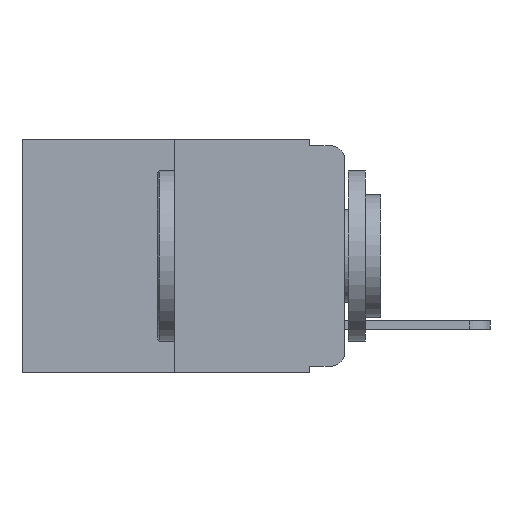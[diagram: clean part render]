
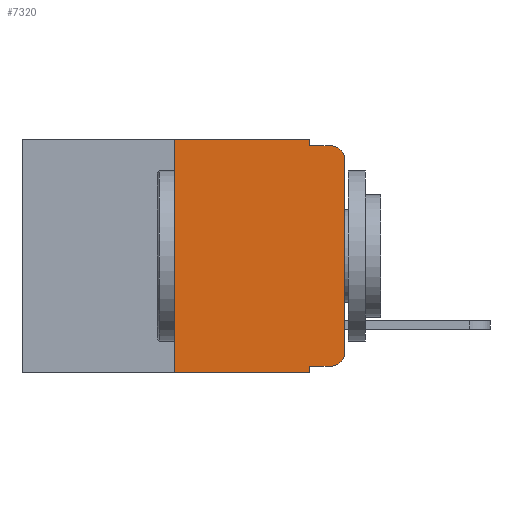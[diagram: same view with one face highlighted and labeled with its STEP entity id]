
A CAD part, left-side view. The second image highlights one B-rep face of the part: STEP entity #7320.
In plain terms, the highlighted planar face has unit normal (-1, 0, 0).
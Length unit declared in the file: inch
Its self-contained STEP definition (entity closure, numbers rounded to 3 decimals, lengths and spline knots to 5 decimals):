
#87 = VECTOR ( 'NONE', #11603, 39.37008 ) ;
#90 = LINE ( 'NONE', #11860, #87 ) ;
#93 = VERTEX_POINT ( 'NONE', #8918 ) ;
#112 = VECTOR ( 'NONE', #10868, 39.37008 ) ;
#142 = VECTOR ( 'NONE', #11367, 39.37008 ) ;
#178 = LINE ( 'NONE', #10943, #112 ) ;
#235 = LINE ( 'NONE', #11436, #142 ) ;
#352 = CIRCLE ( 'NONE', #9233, 0.02 ) ;
#426 = VECTOR ( 'NONE', #11987, 39.37008 ) ;
#482 = CARTESIAN_POINT ( 'NONE',  ( 0., 0.25, -0.343 ) ) ;
#515 = LINE ( 'NONE', #11966, #426 ) ;
#859 = CIRCLE ( 'NONE', #9096, 0.02 ) ;
#1558 = LINE ( 'NONE', #10382, #8378 ) ;
#1566 = VECTOR ( 'NONE', #7424, 39.37008 ) ;
#2270 = EDGE_LOOP ( 'NONE', ( #13273, #12994, #8948, #10997, #10673, #10446, #12246, #12015, #11852, #11502 ) ) ;
#2574 = DIRECTION ( 'NONE',  ( 0., 0., -1. ) ) ;
#2586 = DIRECTION ( 'NONE',  ( 1., 0., 0. ) ) ;
#2614 = CARTESIAN_POINT ( 'NONE',  ( 0., 0.473, 0. ) ) ;
#2624 = PLANE ( 'NONE',  #8270 ) ;
#2682 = DIRECTION ( 'NONE',  ( 0., -1., 0. ) ) ;
#2703 = CARTESIAN_POINT ( 'NONE',  ( 0., 0.473, -0.343 ) ) ;
#2814 = VERTEX_POINT ( 'NONE', #9699 ) ;
#3746 = VECTOR ( 'NONE', #9727, 39.37008 ) ;
#3796 = LINE ( 'NONE', #10735, #3746 ) ;
#3908 = VERTEX_POINT ( 'NONE', #5156 ) ;
#4177 = FACE_OUTER_BOUND ( 'NONE', #2270, .T. ) ;
#5156 = CARTESIAN_POINT ( 'NONE',  ( 0., 0., -0.03 ) ) ;
#5187 = EDGE_CURVE ( 'NONE', #11294, #6536, #3796, .T. ) ;
#6321 = LINE ( 'NONE', #2703, #8980 ) ;
#6351 = CARTESIAN_POINT ( 'NONE',  ( 0., 0., -0.313 ) ) ;
#6403 = VERTEX_POINT ( 'NONE', #12832 ) ;
#6497 = EDGE_CURVE ( 'NONE', #9432, #8527, #515, .T. ) ;
#6517 = EDGE_CURVE ( 'NONE', #8527, #12236, #352, .T. ) ;
#6536 = VERTEX_POINT ( 'NONE', #11826 ) ;
#6566 = EDGE_CURVE ( 'NONE', #9432, #2814, #235, .T. ) ;
#6588 = EDGE_CURVE ( 'NONE', #10835, #11294, #90, .T. ) ;
#6594 = EDGE_CURVE ( 'NONE', #6536, #93, #178, .T. ) ;
#6640 = EDGE_CURVE ( 'NONE', #93, #6403, #1558, .T. ) ;
#6713 = EDGE_CURVE ( 'NONE', #3908, #6403, #859, .T. ) ;
#6931 = EDGE_CURVE ( 'NONE', #12236, #3908, #7455, .T. ) ;
#7309 = EDGE_CURVE ( 'NONE', #10835, #2814, #6321, .T. ) ;
#7320 = ADVANCED_FACE ( 'NONE', ( #4177 ), #2624, .F. ) ;
#7424 = DIRECTION ( 'NONE',  ( 0., 0., 1. ) ) ;
#7455 = LINE ( 'NONE', #7592, #1566 ) ;
#7592 = CARTESIAN_POINT ( 'NONE',  ( 0., 0., 0. ) ) ;
#8270 = AXIS2_PLACEMENT_3D ( 'NONE', #2614, #2586, #2574 ) ;
#8378 = VECTOR ( 'NONE', #10167, 39.37008 ) ;
#8439 = CARTESIAN_POINT ( 'NONE',  ( 0., 0.02, -0.333 ) ) ;
#8527 = VERTEX_POINT ( 'NONE', #8439 ) ;
#8918 = CARTESIAN_POINT ( 'NONE',  ( 0., 0.051, -0.01 ) ) ;
#8948 = ORIENTED_EDGE ( 'NONE', *, *, #6640, .F. ) ;
#8980 = VECTOR ( 'NONE', #2682, 39.37008 ) ;
#9051 = DIRECTION ( 'NONE',  ( 0., 0., -1. ) ) ;
#9063 = DIRECTION ( 'NONE',  ( -1., 0., 0. ) ) ;
#9066 = CARTESIAN_POINT ( 'NONE',  ( 0., 0.02, -0.03 ) ) ;
#9096 = AXIS2_PLACEMENT_3D ( 'NONE', #9066, #9063, #9051 ) ;
#9233 = AXIS2_PLACEMENT_3D ( 'NONE', #11824, #11802, #11734 ) ;
#9432 = VERTEX_POINT ( 'NONE', #12891 ) ;
#9699 = CARTESIAN_POINT ( 'NONE',  ( 0., 0.051, -0.343 ) ) ;
#9727 = DIRECTION ( 'NONE',  ( 0., -1., 0. ) ) ;
#10167 = DIRECTION ( 'NONE',  ( 0., -1., 0. ) ) ;
#10382 = CARTESIAN_POINT ( 'NONE',  ( 0., 0.051, -0.01 ) ) ;
#10446 = ORIENTED_EDGE ( 'NONE', *, *, #6588, .F. ) ;
#10673 = ORIENTED_EDGE ( 'NONE', *, *, #5187, .F. ) ;
#10735 = CARTESIAN_POINT ( 'NONE',  ( 0., 0.473, 0. ) ) ;
#10835 = VERTEX_POINT ( 'NONE', #482 ) ;
#10868 = DIRECTION ( 'NONE',  ( 0., 0., -1. ) ) ;
#10943 = CARTESIAN_POINT ( 'NONE',  ( 0., 0.051, 0. ) ) ;
#10997 = ORIENTED_EDGE ( 'NONE', *, *, #6594, .F. ) ;
#11294 = VERTEX_POINT ( 'NONE', #12195 ) ;
#11367 = DIRECTION ( 'NONE',  ( 0., 0., -1. ) ) ;
#11436 = CARTESIAN_POINT ( 'NONE',  ( 0., 0.051, 0. ) ) ;
#11502 = ORIENTED_EDGE ( 'NONE', *, *, #6517, .T. ) ;
#11603 = DIRECTION ( 'NONE',  ( 0., 0., 1. ) ) ;
#11734 = DIRECTION ( 'NONE',  ( 0., 0., -1. ) ) ;
#11802 = DIRECTION ( 'NONE',  ( -1., 0., 0. ) ) ;
#11824 = CARTESIAN_POINT ( 'NONE',  ( 0., 0.02, -0.313 ) ) ;
#11826 = CARTESIAN_POINT ( 'NONE',  ( 0., 0.051, 0. ) ) ;
#11852 = ORIENTED_EDGE ( 'NONE', *, *, #6497, .T. ) ;
#11860 = CARTESIAN_POINT ( 'NONE',  ( 0., 0.25, 0. ) ) ;
#11966 = CARTESIAN_POINT ( 'NONE',  ( 0., 0.051, -0.333 ) ) ;
#11987 = DIRECTION ( 'NONE',  ( 0., -1., 0. ) ) ;
#12015 = ORIENTED_EDGE ( 'NONE', *, *, #6566, .F. ) ;
#12195 = CARTESIAN_POINT ( 'NONE',  ( 0., 0.25, 0. ) ) ;
#12236 = VERTEX_POINT ( 'NONE', #6351 ) ;
#12246 = ORIENTED_EDGE ( 'NONE', *, *, #7309, .T. ) ;
#12832 = CARTESIAN_POINT ( 'NONE',  ( 0., 0.02, -0.01 ) ) ;
#12891 = CARTESIAN_POINT ( 'NONE',  ( 0., 0.051, -0.333 ) ) ;
#12994 = ORIENTED_EDGE ( 'NONE', *, *, #6713, .T. ) ;
#13273 = ORIENTED_EDGE ( 'NONE', *, *, #6931, .T. ) ;
